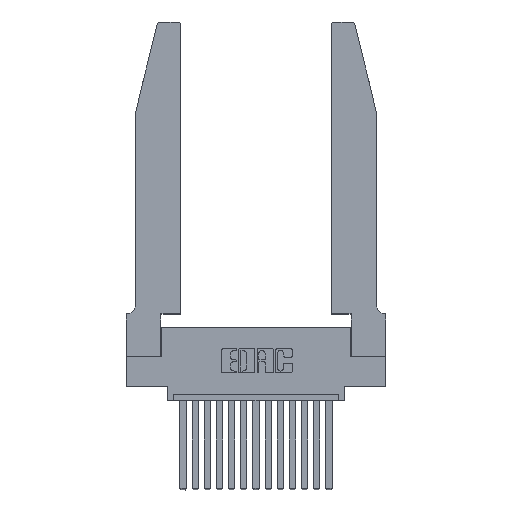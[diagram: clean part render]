
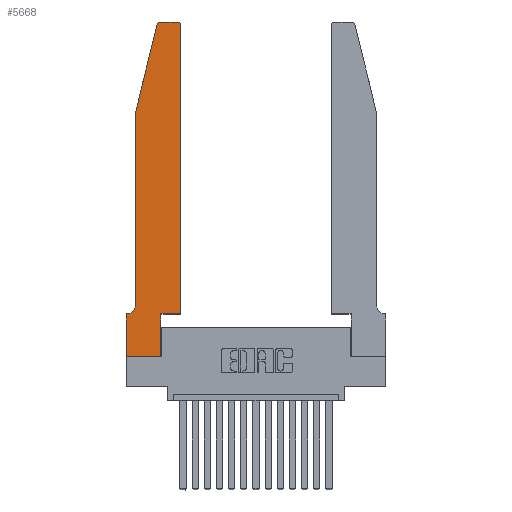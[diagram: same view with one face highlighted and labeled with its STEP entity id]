
A CAD part, top view. The second image highlights one B-rep face of the part: STEP entity #5668.
In plain terms, the highlighted planar face has unit normal (0, 0, 1).
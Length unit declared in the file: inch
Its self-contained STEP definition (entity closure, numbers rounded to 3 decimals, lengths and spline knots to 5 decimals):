
#71 = DIRECTION ( 'NONE',  ( 0., 0., 1. ) ) ;
#93 = ORIENTED_EDGE ( 'NONE', *, *, #5575, .T. ) ;
#100 = EDGE_CURVE ( 'NONE', #2597, #5327, #7076, .T. ) ;
#122 = EDGE_LOOP ( 'NONE', ( #2472, #9632, #12583, #12460, #1210, #14941, #12161, #3149, #13189, #14852, #93, #8103 ) ) ;
#171 = VERTEX_POINT ( 'NONE', #1659 ) ;
#221 = DIRECTION ( 'NONE',  ( -1., 0., 0. ) ) ;
#422 = CARTESIAN_POINT ( 'NONE',  ( 0.2865, 0.35, 0.37 ) ) ;
#626 = VERTEX_POINT ( 'NONE', #947 ) ;
#904 = DIRECTION ( 'NONE',  ( 0., -1., 0. ) ) ;
#947 = CARTESIAN_POINT ( 'NONE',  ( 0.284, 2.75, 0.37 ) ) ;
#969 = CARTESIAN_POINT ( 'NONE',  ( 0.4505, 0.35, 0.37 ) ) ;
#1006 = CARTESIAN_POINT ( 'NONE',  ( 0.0755, 0.42, 0.37 ) ) ;
#1060 = CIRCLE ( 'NONE', #10315, 0.03 ) ;
#1117 = VECTOR ( 'NONE', #11112, 39.37008 ) ;
#1200 = VECTOR ( 'NONE', #10317, 39.37008 ) ;
#1210 = ORIENTED_EDGE ( 'NONE', *, *, #17827, .T. ) ;
#1414 = DIRECTION ( 'NONE',  ( -1., 0., 0. ) ) ;
#1542 = LINE ( 'NONE', #14252, #12432 ) ;
#1659 = CARTESIAN_POINT ( 'NONE',  ( 0.0755, 2., 0.37 ) ) ;
#1945 = VERTEX_POINT ( 'NONE', #10766 ) ;
#2060 = CIRCLE ( 'NONE', #17233, 0.03 ) ;
#2248 = VECTOR ( 'NONE', #15656, 39.37008 ) ;
#2299 = DIRECTION ( 'NONE',  ( 1., 0., 0. ) ) ;
#2316 = VECTOR ( 'NONE', #15644, 39.37008 ) ;
#2454 = VECTOR ( 'NONE', #904, 39.37008 ) ;
#2472 = ORIENTED_EDGE ( 'NONE', *, *, #9975, .T. ) ;
#2589 = CARTESIAN_POINT ( 'NONE',  ( 0.4505, 0.35, 0.37 ) ) ;
#2597 = VERTEX_POINT ( 'NONE', #7922 ) ;
#2801 = CARTESIAN_POINT ( 'NONE',  ( 0.0755, 0.35, 0.37 ) ) ;
#2897 = VERTEX_POINT ( 'NONE', #4396 ) ;
#2909 = LINE ( 'NONE', #12923, #2248 ) ;
#2943 = PLANE ( 'NONE',  #15439 ) ;
#3149 = ORIENTED_EDGE ( 'NONE', *, *, #3598, .T. ) ;
#3273 = CARTESIAN_POINT ( 'NONE',  ( 0., 0.35, 0.37 ) ) ;
#3598 = EDGE_CURVE ( 'NONE', #1945, #2897, #5455, .T. ) ;
#3781 = VERTEX_POINT ( 'NONE', #14909 ) ;
#4396 = CARTESIAN_POINT ( 'NONE',  ( 0.2865, 0., 0.37 ) ) ;
#5327 = VERTEX_POINT ( 'NONE', #3273 ) ;
#5365 = CARTESIAN_POINT ( 'NONE',  ( 0.25487, 2.72718, 0.37 ) ) ;
#5368 = LINE ( 'NONE', #2589, #1117 ) ;
#5455 = LINE ( 'NONE', #7080, #2316 ) ;
#5575 = EDGE_CURVE ( 'NONE', #7861, #9388, #5368, .T. ) ;
#5668 = ADVANCED_FACE ( 'NONE', ( #5808 ), #2943, .T. ) ;
#5684 = EDGE_CURVE ( 'NONE', #16210, #171, #2909, .T. ) ;
#5808 = FACE_OUTER_BOUND ( 'NONE', #122, .T. ) ;
#6006 = VERTEX_POINT ( 'NONE', #1006 ) ;
#6130 = VECTOR ( 'NONE', #9561, 39.37008 ) ;
#6535 = DIRECTION ( 'NONE',  ( 0., 0., -1. ) ) ;
#6666 = VECTOR ( 'NONE', #12647, 39.37008 ) ;
#6912 = LINE ( 'NONE', #7908, #2454 ) ;
#7076 = LINE ( 'NONE', #2801, #7955 ) ;
#7080 = CARTESIAN_POINT ( 'NONE',  ( 0., 0., 0.37 ) ) ;
#7718 = CARTESIAN_POINT ( 'NONE',  ( 0.284, 2.72, 0.37 ) ) ;
#7861 = VERTEX_POINT ( 'NONE', #14757 ) ;
#7908 = CARTESIAN_POINT ( 'NONE',  ( 0., 0., 0.37 ) ) ;
#7922 = CARTESIAN_POINT ( 'NONE',  ( 0.0055, 0.35, 0.37 ) ) ;
#7955 = VECTOR ( 'NONE', #1414, 39.37008 ) ;
#8103 = ORIENTED_EDGE ( 'NONE', *, *, #11241, .T. ) ;
#8502 = EDGE_CURVE ( 'NONE', #171, #6006, #10630, .T. ) ;
#8692 = CARTESIAN_POINT ( 'NONE',  ( 0., 0.35, 0.37 ) ) ;
#9338 = DIRECTION ( 'NONE',  ( 0., 0., 1. ) ) ;
#9388 = VERTEX_POINT ( 'NONE', #11165 ) ;
#9561 = DIRECTION ( 'NONE',  ( 1., 0., 0. ) ) ;
#9632 = ORIENTED_EDGE ( 'NONE', *, *, #14114, .T. ) ;
#9654 = LINE ( 'NONE', #969, #6130 ) ;
#9975 = EDGE_CURVE ( 'NONE', #11988, #626, #1542, .T. ) ;
#10315 = AXIS2_PLACEMENT_3D ( 'NONE', #17718, #9338, #2299 ) ;
#10317 = DIRECTION ( 'NONE',  ( 0., 1., 0. ) ) ;
#10630 = LINE ( 'NONE', #14190, #6666 ) ;
#10712 = DIRECTION ( 'NONE',  ( -1., 0., 0. ) ) ;
#10766 = CARTESIAN_POINT ( 'NONE',  ( 0., 0., 0.37 ) ) ;
#11112 = DIRECTION ( 'NONE',  ( 0., 1., 0. ) ) ;
#11165 = CARTESIAN_POINT ( 'NONE',  ( 0.4505, 2.72, 0.37 ) ) ;
#11241 = EDGE_CURVE ( 'NONE', #9388, #11988, #1060, .T. ) ;
#11447 = AXIS2_PLACEMENT_3D ( 'NONE', #15014, #6535, #10712 ) ;
#11951 = CIRCLE ( 'NONE', #11447, 0.07 ) ;
#11988 = VERTEX_POINT ( 'NONE', #14352 ) ;
#12161 = ORIENTED_EDGE ( 'NONE', *, *, #16688, .T. ) ;
#12374 = EDGE_CURVE ( 'NONE', #3781, #7861, #9654, .T. ) ;
#12432 = VECTOR ( 'NONE', #221, 39.37008 ) ;
#12460 = ORIENTED_EDGE ( 'NONE', *, *, #8502, .T. ) ;
#12583 = ORIENTED_EDGE ( 'NONE', *, *, #5684, .T. ) ;
#12647 = DIRECTION ( 'NONE',  ( 0., -1., 0. ) ) ;
#12923 = CARTESIAN_POINT ( 'NONE',  ( 0.0755, 2., 0.37 ) ) ;
#12986 = DIRECTION ( 'NONE',  ( 1., 0., 0. ) ) ;
#13189 = ORIENTED_EDGE ( 'NONE', *, *, #13682, .T. ) ;
#13682 = EDGE_CURVE ( 'NONE', #2897, #3781, #17393, .T. ) ;
#14114 = EDGE_CURVE ( 'NONE', #626, #16210, #2060, .T. ) ;
#14190 = CARTESIAN_POINT ( 'NONE',  ( 0.0755, 2., 0.37 ) ) ;
#14252 = CARTESIAN_POINT ( 'NONE',  ( 0.2605, 2.75, 0.37 ) ) ;
#14352 = CARTESIAN_POINT ( 'NONE',  ( 0.4205, 2.75, 0.37 ) ) ;
#14757 = CARTESIAN_POINT ( 'NONE',  ( 0.4505, 0.35, 0.37 ) ) ;
#14852 = ORIENTED_EDGE ( 'NONE', *, *, #12374, .T. ) ;
#14909 = CARTESIAN_POINT ( 'NONE',  ( 0.2865, 0.35, 0.37 ) ) ;
#14941 = ORIENTED_EDGE ( 'NONE', *, *, #100, .T. ) ;
#15014 = CARTESIAN_POINT ( 'NONE',  ( 0.0055, 0.42, 0.37 ) ) ;
#15439 = AXIS2_PLACEMENT_3D ( 'NONE', #8692, #71, #17144 ) ;
#15644 = DIRECTION ( 'NONE',  ( 1., 0., 0. ) ) ;
#15656 = DIRECTION ( 'NONE',  ( -0.239, -0.971, 0. ) ) ;
#16210 = VERTEX_POINT ( 'NONE', #5365 ) ;
#16688 = EDGE_CURVE ( 'NONE', #5327, #1945, #6912, .T. ) ;
#17144 = DIRECTION ( 'NONE',  ( 1., 0., 0. ) ) ;
#17233 = AXIS2_PLACEMENT_3D ( 'NONE', #7718, #18119, #12986 ) ;
#17393 = LINE ( 'NONE', #422, #1200 ) ;
#17718 = CARTESIAN_POINT ( 'NONE',  ( 0.4205, 2.72, 0.37 ) ) ;
#17827 = EDGE_CURVE ( 'NONE', #6006, #2597, #11951, .T. ) ;
#18119 = DIRECTION ( 'NONE',  ( 0., 0., 1. ) ) ;
